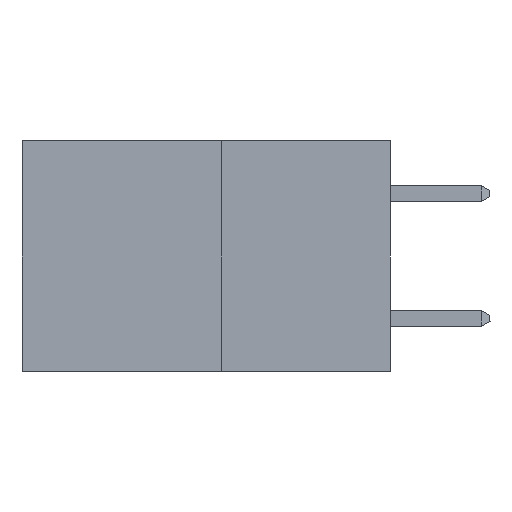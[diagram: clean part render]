
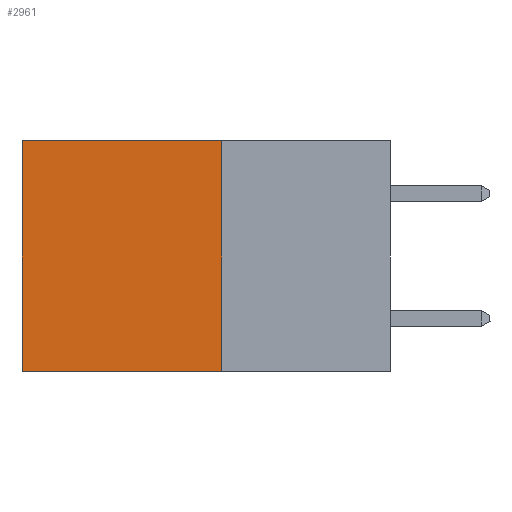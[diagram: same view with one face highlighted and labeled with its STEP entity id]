
A CAD part, left-side view. The second image highlights one B-rep face of the part: STEP entity #2961.
In plain terms, the highlighted planar face has unit normal (-1, 0, 0).
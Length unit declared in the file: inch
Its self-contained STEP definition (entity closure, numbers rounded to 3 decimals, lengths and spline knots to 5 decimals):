
#924 = VERTEX_POINT ( 'NONE', #13392 ) ;
#1003 = CARTESIAN_POINT ( 'NONE',  ( 0.277, 0.27, -0.37 ) ) ;
#2961 = ADVANCED_FACE ( 'NONE', ( #21045 ), #8667, .F. ) ;
#4284 = EDGE_CURVE ( 'NONE', #12846, #30543, #12196, .T. ) ;
#4483 = ORIENTED_EDGE ( 'NONE', *, *, #4284, .F. ) ;
#4835 = VECTOR ( 'NONE', #11325, 39.37008 ) ;
#5339 = CARTESIAN_POINT ( 'NONE',  ( 0.277, 0.27, 0. ) ) ;
#7929 = CARTESIAN_POINT ( 'NONE',  ( 0.277, 0.27, -0.37 ) ) ;
#8633 = DIRECTION ( 'NONE',  ( 0., 0., -1. ) ) ;
#8667 = PLANE ( 'NONE',  #27339 ) ;
#9837 = ORIENTED_EDGE ( 'NONE', *, *, #29555, .T. ) ;
#10024 = CARTESIAN_POINT ( 'NONE',  ( 0.277, 0.27, -0.37 ) ) ;
#10027 = ORIENTED_EDGE ( 'NONE', *, *, #30075, .F. ) ;
#10615 = VECTOR ( 'NONE', #8633, 39.37008 ) ;
#11325 = DIRECTION ( 'NONE',  ( 0., 0., -1. ) ) ;
#12196 = LINE ( 'NONE', #7929, #10615 ) ;
#12846 = VERTEX_POINT ( 'NONE', #17539 ) ;
#13392 = CARTESIAN_POINT ( 'NONE',  ( 0.277, 0.59, -0.37 ) ) ;
#14329 = CARTESIAN_POINT ( 'NONE',  ( 0.277, 0.59, 0. ) ) ;
#17539 = CARTESIAN_POINT ( 'NONE',  ( 0.277, 0.27, 0. ) ) ;
#17976 = DIRECTION ( 'NONE',  ( 0., 1., 0. ) ) ;
#18366 = DIRECTION ( 'NONE',  ( 0., 0., -1. ) ) ;
#18583 = DIRECTION ( 'NONE',  ( 1., 0., 0. ) ) ;
#18733 = VECTOR ( 'NONE', #17976, 39.37008 ) ;
#19747 = EDGE_LOOP ( 'NONE', ( #9837, #10027, #4483, #23411 ) ) ;
#21045 = FACE_OUTER_BOUND ( 'NONE', #19747, .T. ) ;
#21105 = LINE ( 'NONE', #31206, #21867 ) ;
#21867 = VECTOR ( 'NONE', #23709, 39.37008 ) ;
#23411 = ORIENTED_EDGE ( 'NONE', *, *, #29326, .T. ) ;
#23709 = DIRECTION ( 'NONE',  ( 0., 1., 0. ) ) ;
#23802 = VERTEX_POINT ( 'NONE', #14329 ) ;
#27339 = AXIS2_PLACEMENT_3D ( 'NONE', #1003, #18583, #18366 ) ;
#29326 = EDGE_CURVE ( 'NONE', #12846, #23802, #31277, .T. ) ;
#29555 = EDGE_CURVE ( 'NONE', #23802, #924, #30088, .T. ) ;
#30075 = EDGE_CURVE ( 'NONE', #30543, #924, #21105, .T. ) ;
#30088 = LINE ( 'NONE', #31466, #4835 ) ;
#30543 = VERTEX_POINT ( 'NONE', #10024 ) ;
#31206 = CARTESIAN_POINT ( 'NONE',  ( 0.277, 0.27, -0.37 ) ) ;
#31277 = LINE ( 'NONE', #5339, #18733 ) ;
#31466 = CARTESIAN_POINT ( 'NONE',  ( 0.277, 0.59, -0.37 ) ) ;
